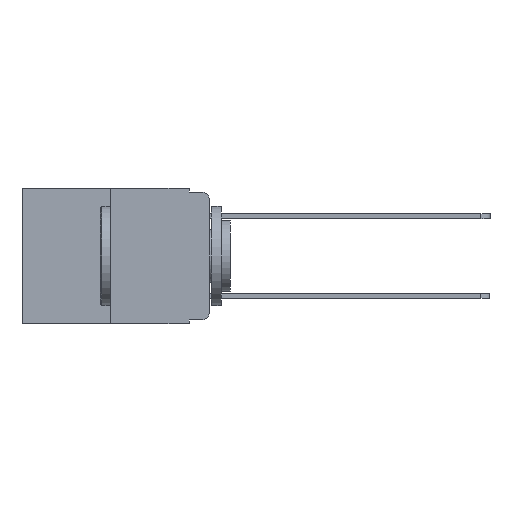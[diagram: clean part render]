
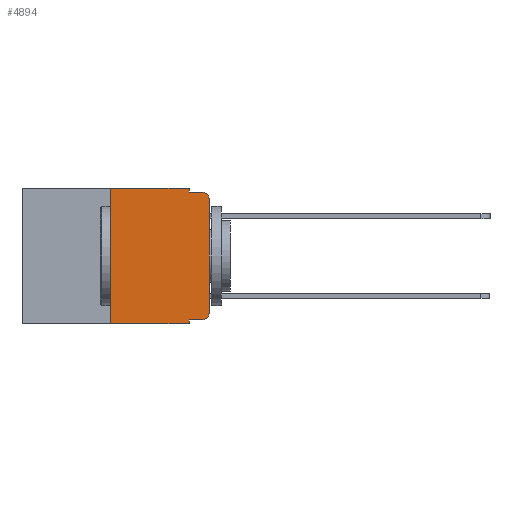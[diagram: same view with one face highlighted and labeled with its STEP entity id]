
A CAD part, left-side view. The second image highlights one B-rep face of the part: STEP entity #4894.
In plain terms, the highlighted planar face has unit normal (-1, 0, 0).
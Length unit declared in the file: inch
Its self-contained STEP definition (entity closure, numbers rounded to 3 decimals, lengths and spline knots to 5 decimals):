
#12 = CARTESIAN_POINT ( 'NONE',  ( 0., 0.051, -0.01 ) ) ;
#18 = DIRECTION ( 'NONE',  ( 0., -1., 0. ) ) ;
#134 = FACE_OUTER_BOUND ( 'NONE', #338, .T. ) ;
#239 = ORIENTED_EDGE ( 'NONE', *, *, #3961, .T. ) ;
#249 = CARTESIAN_POINT ( 'NONE',  ( 0., 0., -0.03 ) ) ;
#282 = LINE ( 'NONE', #4203, #9050 ) ;
#338 = EDGE_LOOP ( 'NONE', ( #8067, #5050, #20024, #19805, #18009, #14727, #12595, #3142, #239, #10961 ) ) ;
#797 = VERTEX_POINT ( 'NONE', #2964 ) ;
#1244 = EDGE_CURVE ( 'NONE', #18594, #797, #15143, .T. ) ;
#1677 = CARTESIAN_POINT ( 'NONE',  ( 0., 0.02, -0.313 ) ) ;
#2042 = VERTEX_POINT ( 'NONE', #249 ) ;
#2192 = PLANE ( 'NONE',  #3923 ) ;
#2360 = VERTEX_POINT ( 'NONE', #15381 ) ;
#2456 = DIRECTION ( 'NONE',  ( 0., 0., -1. ) ) ;
#2543 = VECTOR ( 'NONE', #7466, 39.37008 ) ;
#2896 = AXIS2_PLACEMENT_3D ( 'NONE', #1677, #12881, #3369 ) ;
#2964 = CARTESIAN_POINT ( 'NONE',  ( 0., 0.051, -0.343 ) ) ;
#3036 = VERTEX_POINT ( 'NONE', #6150 ) ;
#3142 = ORIENTED_EDGE ( 'NONE', *, *, #1244, .F. ) ;
#3171 = EDGE_CURVE ( 'NONE', #7156, #3036, #5837, .T. ) ;
#3369 = DIRECTION ( 'NONE',  ( 0., 0., -1. ) ) ;
#3863 = DIRECTION ( 'NONE',  ( 1., 0., 0. ) ) ;
#3923 = AXIS2_PLACEMENT_3D ( 'NONE', #10281, #3863, #14851 ) ;
#3961 = EDGE_CURVE ( 'NONE', #18594, #10651, #282, .T. ) ;
#4066 = VECTOR ( 'NONE', #17465, 39.37008 ) ;
#4203 = CARTESIAN_POINT ( 'NONE',  ( 0., 0.051, -0.333 ) ) ;
#4894 = ADVANCED_FACE ( 'NONE', ( #134 ), #2192, .F. ) ;
#5050 = ORIENTED_EDGE ( 'NONE', *, *, #19765, .T. ) ;
#5291 = EDGE_CURVE ( 'NONE', #16339, #2042, #8372, .T. ) ;
#5435 = EDGE_CURVE ( 'NONE', #8925, #7156, #9613, .T. ) ;
#5837 = LINE ( 'NONE', #18804, #6345 ) ;
#6150 = CARTESIAN_POINT ( 'NONE',  ( 0., 0.051, 0. ) ) ;
#6345 = VECTOR ( 'NONE', #8155, 39.37008 ) ;
#6589 = DIRECTION ( 'NONE',  ( 0., -1., 0. ) ) ;
#7156 = VERTEX_POINT ( 'NONE', #14251 ) ;
#7206 = EDGE_CURVE ( 'NONE', #7237, #2360, #20182, .T. ) ;
#7237 = VERTEX_POINT ( 'NONE', #12 ) ;
#7466 = DIRECTION ( 'NONE',  ( 0., 0., -1. ) ) ;
#8067 = ORIENTED_EDGE ( 'NONE', *, *, #5291, .T. ) ;
#8155 = DIRECTION ( 'NONE',  ( 0., -1., 0. ) ) ;
#8236 = DIRECTION ( 'NONE',  ( -1., 0., 0. ) ) ;
#8306 = CARTESIAN_POINT ( 'NONE',  ( 0., 0., 0. ) ) ;
#8372 = LINE ( 'NONE', #8306, #4066 ) ;
#8532 = VECTOR ( 'NONE', #6589, 39.37008 ) ;
#8654 = CARTESIAN_POINT ( 'NONE',  ( 0., 0.25, 0. ) ) ;
#8925 = VERTEX_POINT ( 'NONE', #20095 ) ;
#9050 = VECTOR ( 'NONE', #16765, 39.37008 ) ;
#9129 = LINE ( 'NONE', #15984, #16776 ) ;
#9613 = LINE ( 'NONE', #8654, #10107 ) ;
#9650 = LINE ( 'NONE', #12039, #17707 ) ;
#10107 = VECTOR ( 'NONE', #17781, 39.37008 ) ;
#10281 = CARTESIAN_POINT ( 'NONE',  ( 0., 0.473, 0. ) ) ;
#10302 = CIRCLE ( 'NONE', #2896, 0.02 ) ;
#10651 = VERTEX_POINT ( 'NONE', #18877 ) ;
#10961 = ORIENTED_EDGE ( 'NONE', *, *, #11293, .T. ) ;
#11293 = EDGE_CURVE ( 'NONE', #10651, #16339, #10302, .T. ) ;
#12039 = CARTESIAN_POINT ( 'NONE',  ( 0., 0.051, 0. ) ) ;
#12595 = ORIENTED_EDGE ( 'NONE', *, *, #17392, .T. ) ;
#12881 = DIRECTION ( 'NONE',  ( -1., 0., 0. ) ) ;
#13369 = CARTESIAN_POINT ( 'NONE',  ( 0., 0., -0.313 ) ) ;
#14251 = CARTESIAN_POINT ( 'NONE',  ( 0., 0.25, 0. ) ) ;
#14727 = ORIENTED_EDGE ( 'NONE', *, *, #5435, .F. ) ;
#14851 = DIRECTION ( 'NONE',  ( 0., 0., -1. ) ) ;
#15143 = LINE ( 'NONE', #16691, #2543 ) ;
#15381 = CARTESIAN_POINT ( 'NONE',  ( 0., 0.02, -0.01 ) ) ;
#15858 = EDGE_CURVE ( 'NONE', #3036, #7237, #9650, .T. ) ;
#15984 = CARTESIAN_POINT ( 'NONE',  ( 0., 0.473, -0.343 ) ) ;
#16339 = VERTEX_POINT ( 'NONE', #13369 ) ;
#16691 = CARTESIAN_POINT ( 'NONE',  ( 0., 0.051, 0. ) ) ;
#16765 = DIRECTION ( 'NONE',  ( 0., -1., 0. ) ) ;
#16776 = VECTOR ( 'NONE', #18, 39.37008 ) ;
#17346 = CARTESIAN_POINT ( 'NONE',  ( 0., 0.051, -0.01 ) ) ;
#17392 = EDGE_CURVE ( 'NONE', #8925, #797, #9129, .T. ) ;
#17397 = CARTESIAN_POINT ( 'NONE',  ( 0., 0.02, -0.03 ) ) ;
#17434 = CARTESIAN_POINT ( 'NONE',  ( 0., 0.051, -0.333 ) ) ;
#17465 = DIRECTION ( 'NONE',  ( 0., 0., 1. ) ) ;
#17707 = VECTOR ( 'NONE', #2456, 39.37008 ) ;
#17781 = DIRECTION ( 'NONE',  ( 0., 0., 1. ) ) ;
#18009 = ORIENTED_EDGE ( 'NONE', *, *, #3171, .F. ) ;
#18296 = AXIS2_PLACEMENT_3D ( 'NONE', #17397, #8236, #18887 ) ;
#18594 = VERTEX_POINT ( 'NONE', #17434 ) ;
#18804 = CARTESIAN_POINT ( 'NONE',  ( 0., 0.473, 0. ) ) ;
#18877 = CARTESIAN_POINT ( 'NONE',  ( 0., 0.02, -0.333 ) ) ;
#18887 = DIRECTION ( 'NONE',  ( 0., 0., -1. ) ) ;
#19490 = CIRCLE ( 'NONE', #18296, 0.02 ) ;
#19765 = EDGE_CURVE ( 'NONE', #2042, #2360, #19490, .T. ) ;
#19805 = ORIENTED_EDGE ( 'NONE', *, *, #15858, .F. ) ;
#20024 = ORIENTED_EDGE ( 'NONE', *, *, #7206, .F. ) ;
#20095 = CARTESIAN_POINT ( 'NONE',  ( 0., 0.25, -0.343 ) ) ;
#20182 = LINE ( 'NONE', #17346, #8532 ) ;
